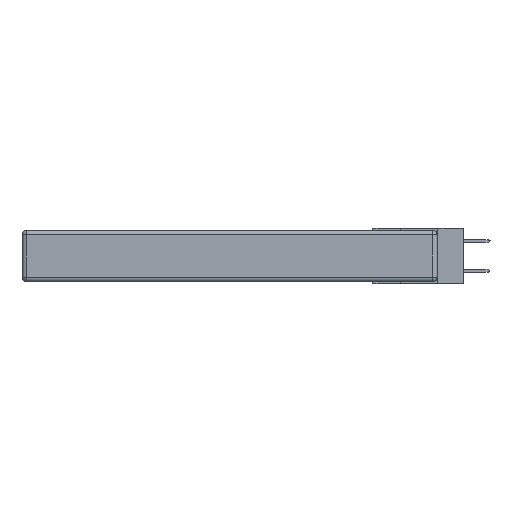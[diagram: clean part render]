
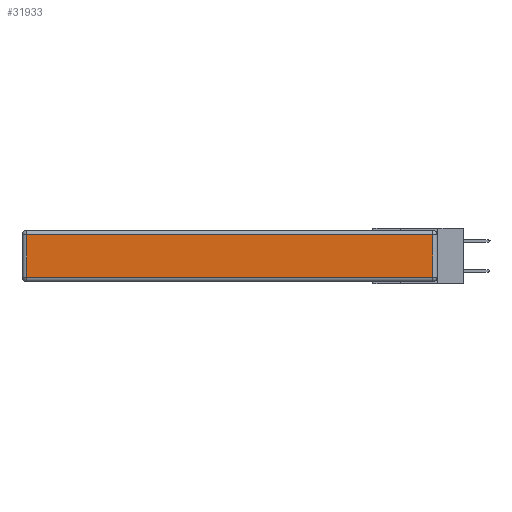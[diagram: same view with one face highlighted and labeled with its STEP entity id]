
A CAD part, left-side view. The second image highlights one B-rep face of the part: STEP entity #31933.
In plain terms, the highlighted planar face has unit normal (-1, 0, 0).
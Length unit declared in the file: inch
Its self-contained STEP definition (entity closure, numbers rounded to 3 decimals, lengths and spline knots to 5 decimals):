
#456 = VERTEX_POINT ( 'NONE', #22900 ) ;
#861 = CARTESIAN_POINT ( 'NONE',  ( 0., 0., -0.343 ) ) ;
#3379 = VECTOR ( 'NONE', #32930, 39.37008 ) ;
#3592 = CARTESIAN_POINT ( 'NONE',  ( 0., 2.75, -0.03 ) ) ;
#4492 = CARTESIAN_POINT ( 'NONE',  ( 0., 0.03, -0.03 ) ) ;
#5283 = EDGE_CURVE ( 'NONE', #13626, #456, #22877, .T. ) ;
#5992 = DIRECTION ( 'NONE',  ( -1., 0., 0. ) ) ;
#7244 = EDGE_CURVE ( 'NONE', #456, #32515, #28799, .T. ) ;
#8704 = CARTESIAN_POINT ( 'NONE',  ( 0., 2.72, -0.313 ) ) ;
#9018 = EDGE_LOOP ( 'NONE', ( #28954, #11443, #9222, #18754 ) ) ;
#9222 = ORIENTED_EDGE ( 'NONE', *, *, #23929, .T. ) ;
#9897 = CARTESIAN_POINT ( 'NONE',  ( 0., 2.72, -0.03 ) ) ;
#11443 = ORIENTED_EDGE ( 'NONE', *, *, #7244, .T. ) ;
#12227 = FACE_OUTER_BOUND ( 'NONE', #9018, .T. ) ;
#12289 = VECTOR ( 'NONE', #14523, 39.37008 ) ;
#12296 = EDGE_CURVE ( 'NONE', #19587, #13626, #23431, .T. ) ;
#13626 = VERTEX_POINT ( 'NONE', #8704 ) ;
#13683 = DIRECTION ( 'NONE',  ( 0., 0., 1. ) ) ;
#14523 = DIRECTION ( 'NONE',  ( 0., 0., -1. ) ) ;
#15227 = VECTOR ( 'NONE', #18718, 39.37008 ) ;
#15964 = CARTESIAN_POINT ( 'NONE',  ( 0., 0.03, -0.343 ) ) ;
#18486 = VECTOR ( 'NONE', #18712, 39.37008 ) ;
#18712 = DIRECTION ( 'NONE',  ( 0., 1., 0. ) ) ;
#18718 = DIRECTION ( 'NONE',  ( 0., 0., 1. ) ) ;
#18754 = ORIENTED_EDGE ( 'NONE', *, *, #12296, .T. ) ;
#19587 = VERTEX_POINT ( 'NONE', #9897 ) ;
#21608 = CARTESIAN_POINT ( 'NONE',  ( 0., 2.72, -0.343 ) ) ;
#22877 = LINE ( 'NONE', #28060, #3379 ) ;
#22900 = CARTESIAN_POINT ( 'NONE',  ( 0., 0.03, -0.313 ) ) ;
#23431 = LINE ( 'NONE', #21608, #12289 ) ;
#23929 = EDGE_CURVE ( 'NONE', #32515, #19587, #30475, .T. ) ;
#25881 = AXIS2_PLACEMENT_3D ( 'NONE', #861, #5992, #13683 ) ;
#28060 = CARTESIAN_POINT ( 'NONE',  ( 0., 0., -0.313 ) ) ;
#28799 = LINE ( 'NONE', #15964, #15227 ) ;
#28954 = ORIENTED_EDGE ( 'NONE', *, *, #5283, .T. ) ;
#29274 = PLANE ( 'NONE',  #25881 ) ;
#30475 = LINE ( 'NONE', #3592, #18486 ) ;
#31933 = ADVANCED_FACE ( 'NONE', ( #12227 ), #29274, .T. ) ;
#32515 = VERTEX_POINT ( 'NONE', #4492 ) ;
#32930 = DIRECTION ( 'NONE',  ( 0., -1., 0. ) ) ;
